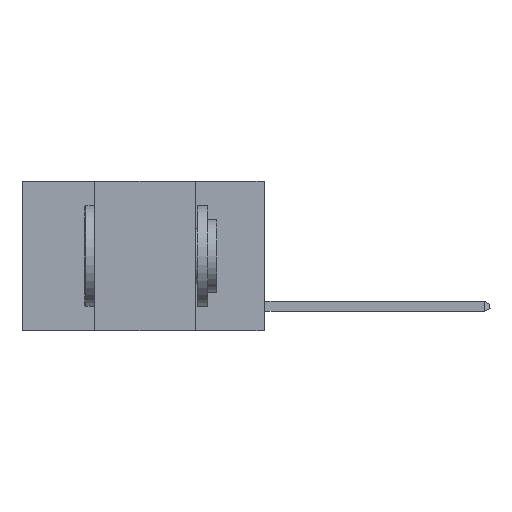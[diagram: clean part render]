
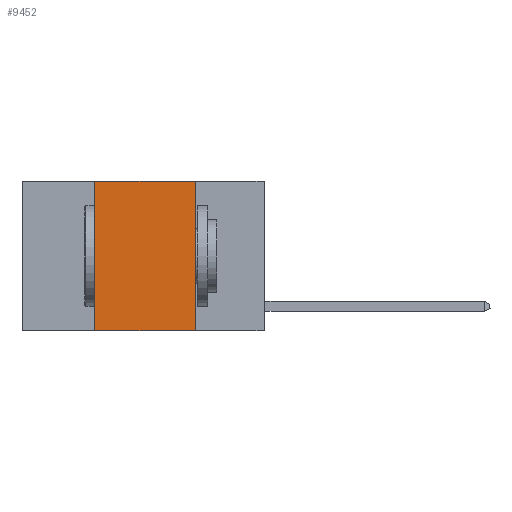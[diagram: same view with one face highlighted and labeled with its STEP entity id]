
A CAD part, left-side view. The second image highlights one B-rep face of the part: STEP entity #9452.
In plain terms, the highlighted planar face has unit normal (-1, 0, 0).
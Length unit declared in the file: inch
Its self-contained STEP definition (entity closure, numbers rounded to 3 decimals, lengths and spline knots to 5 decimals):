
#92 = VERTEX_POINT ( 'NONE', #2919 ) ;
#1088 = PLANE ( 'NONE',  #10625 ) ;
#1871 = VECTOR ( 'NONE', #13754, 39.37008 ) ;
#2487 = ORIENTED_EDGE ( 'NONE', *, *, #4321, .T. ) ;
#2919 = CARTESIAN_POINT ( 'NONE',  ( 0., 0.17, -0.37 ) ) ;
#4321 = EDGE_CURVE ( 'NONE', #15785, #92, #13726, .T. ) ;
#6049 = LINE ( 'NONE', #15596, #7545 ) ;
#6067 = EDGE_CURVE ( 'NONE', #6218, #10295, #6049, .T. ) ;
#6218 = VERTEX_POINT ( 'NONE', #14753 ) ;
#7293 = CARTESIAN_POINT ( 'NONE',  ( 0., 0.42, 0. ) ) ;
#7545 = VECTOR ( 'NONE', #12508, 39.37008 ) ;
#8806 = DIRECTION ( 'NONE',  ( 0., 0., -1. ) ) ;
#9452 = ADVANCED_FACE ( 'NONE', ( #18707 ), #1088, .F. ) ;
#10295 = VERTEX_POINT ( 'NONE', #14270 ) ;
#10400 = LINE ( 'NONE', #16962, #16694 ) ;
#10622 = DIRECTION ( 'NONE',  ( 0., 0., -1. ) ) ;
#10624 = DIRECTION ( 'NONE',  ( 0., -1., 0. ) ) ;
#10625 = AXIS2_PLACEMENT_3D ( 'NONE', #14138, #20617, #10622 ) ;
#10668 = ORIENTED_EDGE ( 'NONE', *, *, #6067, .F. ) ;
#12149 = LINE ( 'NONE', #7293, #1871 ) ;
#12508 = DIRECTION ( 'NONE',  ( 0., -1., 0. ) ) ;
#12511 = VECTOR ( 'NONE', #10624, 39.37008 ) ;
#13647 = EDGE_CURVE ( 'NONE', #10295, #92, #10400, .T. ) ;
#13726 = LINE ( 'NONE', #15617, #12511 ) ;
#13754 = DIRECTION ( 'NONE',  ( 0., 0., 1. ) ) ;
#14138 = CARTESIAN_POINT ( 'NONE',  ( 0., 0.6, 0. ) ) ;
#14270 = CARTESIAN_POINT ( 'NONE',  ( 0., 0.17, 0. ) ) ;
#14612 = CARTESIAN_POINT ( 'NONE',  ( 0., 0.42, -0.37 ) ) ;
#14753 = CARTESIAN_POINT ( 'NONE',  ( 0., 0.42, 0. ) ) ;
#15596 = CARTESIAN_POINT ( 'NONE',  ( 0., 0.6, 0. ) ) ;
#15617 = CARTESIAN_POINT ( 'NONE',  ( 0., 0.6, -0.37 ) ) ;
#15785 = VERTEX_POINT ( 'NONE', #14612 ) ;
#15840 = EDGE_CURVE ( 'NONE', #15785, #6218, #12149, .T. ) ;
#16694 = VECTOR ( 'NONE', #8806, 39.37008 ) ;
#16962 = CARTESIAN_POINT ( 'NONE',  ( 0., 0.17, 0. ) ) ;
#17107 = ORIENTED_EDGE ( 'NONE', *, *, #13647, .F. ) ;
#18707 = FACE_OUTER_BOUND ( 'NONE', #20191, .T. ) ;
#20104 = ORIENTED_EDGE ( 'NONE', *, *, #15840, .F. ) ;
#20191 = EDGE_LOOP ( 'NONE', ( #17107, #10668, #20104, #2487 ) ) ;
#20617 = DIRECTION ( 'NONE',  ( 1., 0., 0. ) ) ;
